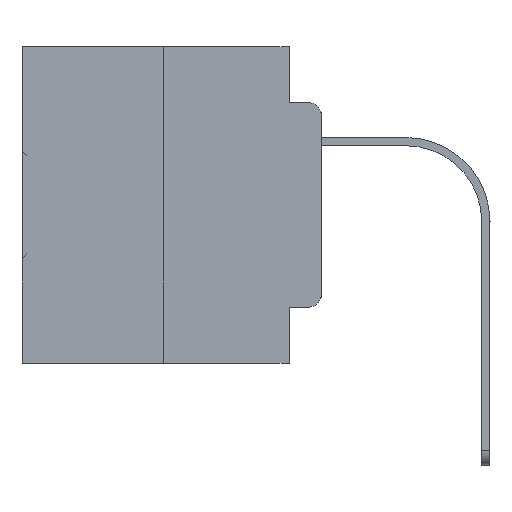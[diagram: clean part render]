
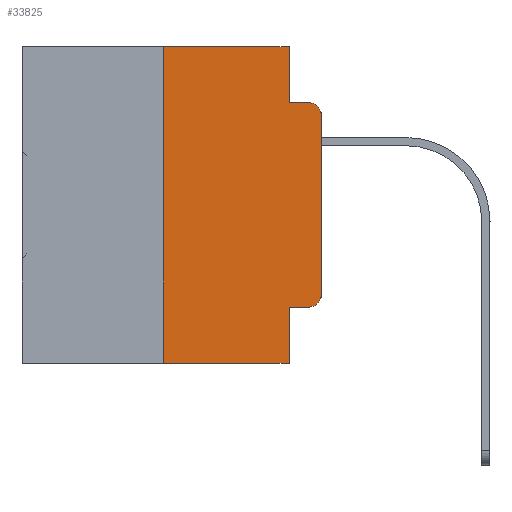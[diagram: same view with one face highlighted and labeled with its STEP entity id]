
A CAD part, left-side view. The second image highlights one B-rep face of the part: STEP entity #33825.
In plain terms, the highlighted planar face has unit normal (-1, 0, 0).
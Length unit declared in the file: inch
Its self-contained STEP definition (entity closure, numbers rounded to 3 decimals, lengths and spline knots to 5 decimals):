
#289 = DIRECTION ( 'NONE',  ( 0., -1., 0. ) ) ;
#367 = VERTEX_POINT ( 'NONE', #33907 ) ;
#493 = ORIENTED_EDGE ( 'NONE', *, *, #25069, .T. ) ;
#514 = EDGE_CURVE ( 'NONE', #13079, #21242, #22736, .T. ) ;
#806 = CARTESIAN_POINT ( 'NONE',  ( 0., 0.473, 0. ) ) ;
#924 = VERTEX_POINT ( 'NONE', #11214 ) ;
#1257 = AXIS2_PLACEMENT_3D ( 'NONE', #18500, #13013, #15900 ) ;
#1770 = DIRECTION ( 'NONE',  ( 0., -1., 0. ) ) ;
#1892 = VERTEX_POINT ( 'NONE', #28057 ) ;
#2242 = CARTESIAN_POINT ( 'NONE',  ( 0., 0., -0.3915 ) ) ;
#2354 = ORIENTED_EDGE ( 'NONE', *, *, #26744, .F. ) ;
#2522 = CARTESIAN_POINT ( 'NONE',  ( 0., 0., -0.1085 ) ) ;
#2807 = DIRECTION ( 'NONE',  ( 0., -1., 0. ) ) ;
#2879 = DIRECTION ( 'NONE',  ( -1., 0., 0. ) ) ;
#4480 = EDGE_CURVE ( 'NONE', #7106, #924, #21009, .T. ) ;
#5767 = VECTOR ( 'NONE', #18365, 39.37008 ) ;
#6548 = ORIENTED_EDGE ( 'NONE', *, *, #14854, .T. ) ;
#6953 = VECTOR ( 'NONE', #27412, 39.37008 ) ;
#7106 = VERTEX_POINT ( 'NONE', #2522 ) ;
#7529 = CARTESIAN_POINT ( 'NONE',  ( 0., 0.25, 0. ) ) ;
#7990 = ORIENTED_EDGE ( 'NONE', *, *, #26483, .T. ) ;
#8232 = LINE ( 'NONE', #26234, #31176 ) ;
#9239 = DIRECTION ( 'NONE',  ( 1., 0., 0. ) ) ;
#9599 = CARTESIAN_POINT ( 'NONE',  ( 0., 0.473, 0. ) ) ;
#10553 = CARTESIAN_POINT ( 'NONE',  ( 0., 0.051, -0.0885 ) ) ;
#11214 = CARTESIAN_POINT ( 'NONE',  ( 0., 0.02, -0.0885 ) ) ;
#11622 = EDGE_CURVE ( 'NONE', #21242, #12492, #8232, .T. ) ;
#12492 = VERTEX_POINT ( 'NONE', #13258 ) ;
#12591 = EDGE_LOOP ( 'NONE', ( #493, #14121, #31346, #13945, #14770, #20646, #7990, #2354, #6548, #14758 ) ) ;
#13009 = LINE ( 'NONE', #28749, #23535 ) ;
#13013 = DIRECTION ( 'NONE',  ( -1., 0., 0. ) ) ;
#13030 = CARTESIAN_POINT ( 'NONE',  ( 0., 0.473, -0.5 ) ) ;
#13079 = VERTEX_POINT ( 'NONE', #7529 ) ;
#13258 = CARTESIAN_POINT ( 'NONE',  ( 0., 0.051, -0.0885 ) ) ;
#13734 = CARTESIAN_POINT ( 'NONE',  ( 0., 0.051, -0.4115 ) ) ;
#13945 = ORIENTED_EDGE ( 'NONE', *, *, #11622, .F. ) ;
#14121 = ORIENTED_EDGE ( 'NONE', *, *, #4480, .T. ) ;
#14403 = PLANE ( 'NONE',  #33401 ) ;
#14552 = CARTESIAN_POINT ( 'NONE',  ( 0., 0.051, 0. ) ) ;
#14758 = ORIENTED_EDGE ( 'NONE', *, *, #23773, .T. ) ;
#14770 = ORIENTED_EDGE ( 'NONE', *, *, #514, .F. ) ;
#14854 = EDGE_CURVE ( 'NONE', #27807, #367, #20363, .T. ) ;
#14899 = FACE_OUTER_BOUND ( 'NONE', #12591, .T. ) ;
#15426 = DIRECTION ( 'NONE',  ( 0., 0., -1. ) ) ;
#15900 = DIRECTION ( 'NONE',  ( 0., 0., -1. ) ) ;
#16379 = LINE ( 'NONE', #10553, #20534 ) ;
#16661 = VECTOR ( 'NONE', #1770, 39.37008 ) ;
#17811 = DIRECTION ( 'NONE',  ( 0., 0., 1. ) ) ;
#18188 = LINE ( 'NONE', #31680, #5767 ) ;
#18365 = DIRECTION ( 'NONE',  ( 0., 0., 1. ) ) ;
#18500 = CARTESIAN_POINT ( 'NONE',  ( 0., 0.02, -0.1085 ) ) ;
#18850 = CIRCLE ( 'NONE', #22117, 0.02 ) ;
#20013 = EDGE_CURVE ( 'NONE', #12492, #924, #16379, .T. ) ;
#20077 = DIRECTION ( 'NONE',  ( 0., 0., -1. ) ) ;
#20363 = LINE ( 'NONE', #22445, #6953 ) ;
#20534 = VECTOR ( 'NONE', #2807, 39.37008 ) ;
#20646 = ORIENTED_EDGE ( 'NONE', *, *, #28171, .F. ) ;
#21009 = CIRCLE ( 'NONE', #1257, 0.02 ) ;
#21092 = CARTESIAN_POINT ( 'NONE',  ( 0., 0.02, -0.3915 ) ) ;
#21242 = VERTEX_POINT ( 'NONE', #23931 ) ;
#22117 = AXIS2_PLACEMENT_3D ( 'NONE', #21092, #2879, #15426 ) ;
#22445 = CARTESIAN_POINT ( 'NONE',  ( 0., 0.051, -0.4115 ) ) ;
#22736 = LINE ( 'NONE', #806, #16661 ) ;
#23535 = VECTOR ( 'NONE', #17811, 39.37008 ) ;
#23773 = EDGE_CURVE ( 'NONE', #367, #28995, #18850, .T. ) ;
#23931 = CARTESIAN_POINT ( 'NONE',  ( 0., 0.051, 0. ) ) ;
#24820 = DIRECTION ( 'NONE',  ( 0., 0., -1. ) ) ;
#25069 = EDGE_CURVE ( 'NONE', #28995, #7106, #18188, .T. ) ;
#25613 = VERTEX_POINT ( 'NONE', #33713 ) ;
#26234 = CARTESIAN_POINT ( 'NONE',  ( 0., 0.051, 0. ) ) ;
#26483 = EDGE_CURVE ( 'NONE', #25613, #1892, #31513, .T. ) ;
#26569 = VECTOR ( 'NONE', #24820, 39.37008 ) ;
#26744 = EDGE_CURVE ( 'NONE', #27807, #1892, #27558, .T. ) ;
#27412 = DIRECTION ( 'NONE',  ( 0., -1., 0. ) ) ;
#27558 = LINE ( 'NONE', #14552, #26569 ) ;
#27807 = VERTEX_POINT ( 'NONE', #13734 ) ;
#28057 = CARTESIAN_POINT ( 'NONE',  ( 0., 0.051, -0.5 ) ) ;
#28171 = EDGE_CURVE ( 'NONE', #25613, #13079, #13009, .T. ) ;
#28749 = CARTESIAN_POINT ( 'NONE',  ( 0., 0.25, 0. ) ) ;
#28995 = VERTEX_POINT ( 'NONE', #2242 ) ;
#30387 = VECTOR ( 'NONE', #289, 39.37008 ) ;
#31176 = VECTOR ( 'NONE', #31538, 39.37008 ) ;
#31346 = ORIENTED_EDGE ( 'NONE', *, *, #20013, .F. ) ;
#31513 = LINE ( 'NONE', #13030, #30387 ) ;
#31538 = DIRECTION ( 'NONE',  ( 0., 0., -1. ) ) ;
#31680 = CARTESIAN_POINT ( 'NONE',  ( 0., 0., 0. ) ) ;
#33401 = AXIS2_PLACEMENT_3D ( 'NONE', #9599, #9239, #20077 ) ;
#33713 = CARTESIAN_POINT ( 'NONE',  ( 0., 0.25, -0.5 ) ) ;
#33825 = ADVANCED_FACE ( 'NONE', ( #14899 ), #14403, .F. ) ;
#33907 = CARTESIAN_POINT ( 'NONE',  ( 0., 0.02, -0.4115 ) ) ;
